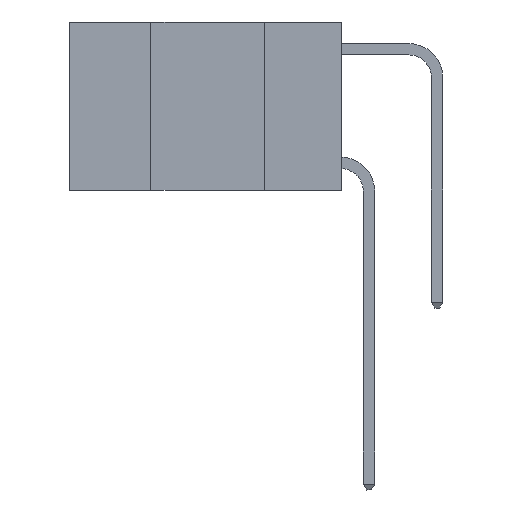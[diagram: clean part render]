
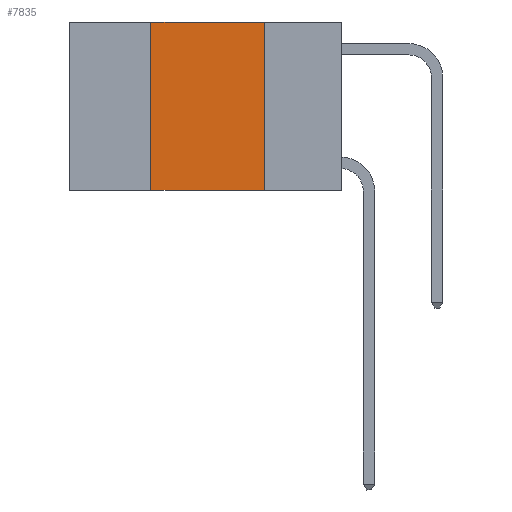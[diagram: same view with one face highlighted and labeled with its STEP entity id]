
A CAD part, left-side view. The second image highlights one B-rep face of the part: STEP entity #7835.
In plain terms, the highlighted planar face has unit normal (-1, 0, 0).
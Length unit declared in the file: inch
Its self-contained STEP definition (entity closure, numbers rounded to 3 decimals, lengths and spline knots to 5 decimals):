
#84 = LINE ( 'NONE', #7047, #3389 ) ;
#487 = ORIENTED_EDGE ( 'NONE', *, *, #9794, .T. ) ;
#660 = EDGE_LOOP ( 'NONE', ( #9506, #9225, #5877, #487 ) ) ;
#893 = VERTEX_POINT ( 'NONE', #7656 ) ;
#1186 = CARTESIAN_POINT ( 'NONE',  ( 0., 0.6, -0.37 ) ) ;
#1542 = CARTESIAN_POINT ( 'NONE',  ( 0., 0.6, 0. ) ) ;
#1771 = AXIS2_PLACEMENT_3D ( 'NONE', #9896, #6183, #10660 ) ;
#2326 = CARTESIAN_POINT ( 'NONE',  ( 0., 0.17, -0.37 ) ) ;
#3343 = CARTESIAN_POINT ( 'NONE',  ( 0., 0.42, 0. ) ) ;
#3357 = DIRECTION ( 'NONE',  ( 0., -1., 0. ) ) ;
#3389 = VECTOR ( 'NONE', #5212, 39.37008 ) ;
#3432 = VECTOR ( 'NONE', #6472, 39.37008 ) ;
#4332 = EDGE_CURVE ( 'NONE', #893, #10047, #84, .T. ) ;
#4572 = LINE ( 'NONE', #8037, #3432 ) ;
#4701 = DIRECTION ( 'NONE',  ( 0., -1., 0. ) ) ;
#5212 = DIRECTION ( 'NONE',  ( 0., 0., 1. ) ) ;
#5588 = CARTESIAN_POINT ( 'NONE',  ( 0., 0.17, 0. ) ) ;
#5628 = LINE ( 'NONE', #1186, #10788 ) ;
#5877 = ORIENTED_EDGE ( 'NONE', *, *, #4332, .F. ) ;
#6183 = DIRECTION ( 'NONE',  ( 1., 0., 0. ) ) ;
#6472 = DIRECTION ( 'NONE',  ( 0., 0., -1. ) ) ;
#7047 = CARTESIAN_POINT ( 'NONE',  ( 0., 0.42, 0. ) ) ;
#7103 = VECTOR ( 'NONE', #3357, 39.37008 ) ;
#7148 = PLANE ( 'NONE',  #1771 ) ;
#7413 = EDGE_CURVE ( 'NONE', #9299, #9115, #4572, .T. ) ;
#7656 = CARTESIAN_POINT ( 'NONE',  ( 0., 0.42, -0.37 ) ) ;
#7835 = ADVANCED_FACE ( 'NONE', ( #8987 ), #7148, .F. ) ;
#8037 = CARTESIAN_POINT ( 'NONE',  ( 0., 0.17, 0. ) ) ;
#8987 = FACE_OUTER_BOUND ( 'NONE', #660, .T. ) ;
#9115 = VERTEX_POINT ( 'NONE', #2326 ) ;
#9225 = ORIENTED_EDGE ( 'NONE', *, *, #9517, .F. ) ;
#9299 = VERTEX_POINT ( 'NONE', #5588 ) ;
#9506 = ORIENTED_EDGE ( 'NONE', *, *, #7413, .F. ) ;
#9517 = EDGE_CURVE ( 'NONE', #10047, #9299, #10239, .T. ) ;
#9794 = EDGE_CURVE ( 'NONE', #893, #9115, #5628, .T. ) ;
#9896 = CARTESIAN_POINT ( 'NONE',  ( 0., 0.6, 0. ) ) ;
#10047 = VERTEX_POINT ( 'NONE', #3343 ) ;
#10239 = LINE ( 'NONE', #1542, #7103 ) ;
#10660 = DIRECTION ( 'NONE',  ( 0., 0., -1. ) ) ;
#10788 = VECTOR ( 'NONE', #4701, 39.37008 ) ;
